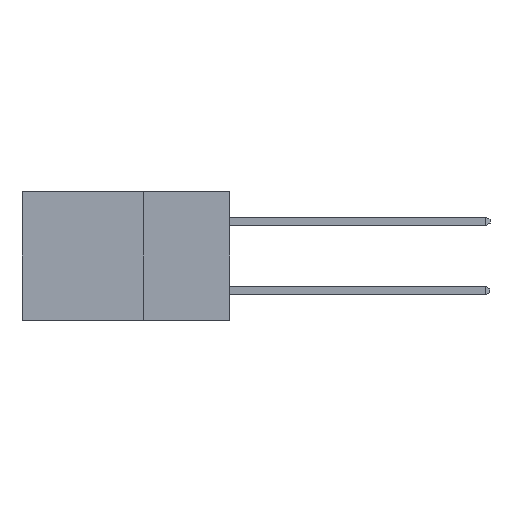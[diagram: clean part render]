
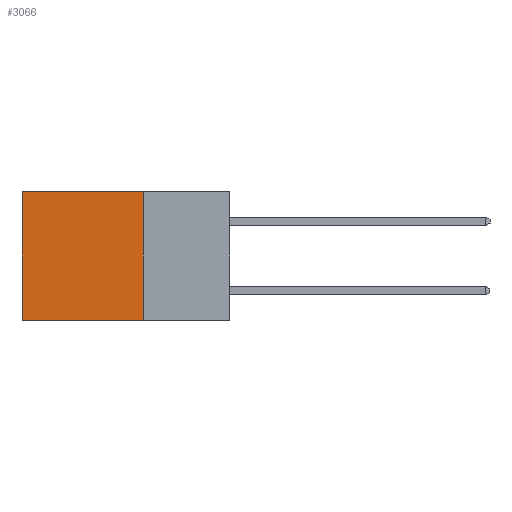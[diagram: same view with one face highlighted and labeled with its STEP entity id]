
A CAD part, left-side view. The second image highlights one B-rep face of the part: STEP entity #3066.
In plain terms, the highlighted planar face has unit normal (-1, 0, 0).
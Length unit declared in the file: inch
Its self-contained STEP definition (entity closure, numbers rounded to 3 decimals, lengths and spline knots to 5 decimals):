
#814 = AXIS2_PLACEMENT_3D ( 'NONE', #14183, #15251, #17469 ) ;
#2718 = VECTOR ( 'NONE', #5513, 39.37008 ) ;
#3066 = ADVANCED_FACE ( 'NONE', ( #17474 ), #12398, .F. ) ;
#3145 = VECTOR ( 'NONE', #8447, 39.37008 ) ;
#3818 = EDGE_CURVE ( 'NONE', #6233, #23538, #18302, .T. ) ;
#4454 = EDGE_CURVE ( 'NONE', #7965, #6233, #12601, .T. ) ;
#5513 = DIRECTION ( 'NONE',  ( 0., 0., -1. ) ) ;
#6233 = VERTEX_POINT ( 'NONE', #17590 ) ;
#7965 = VERTEX_POINT ( 'NONE', #8182 ) ;
#8182 = CARTESIAN_POINT ( 'NONE',  ( 0.298, 0.25, 0. ) ) ;
#8401 = ORIENTED_EDGE ( 'NONE', *, *, #19757, .F. ) ;
#8447 = DIRECTION ( 'NONE',  ( 0., 0., -1. ) ) ;
#8941 = EDGE_LOOP ( 'NONE', ( #13513, #8401, #20923, #21723 ) ) ;
#8965 = LINE ( 'NONE', #9352, #13860 ) ;
#9352 = CARTESIAN_POINT ( 'NONE',  ( 0.298, 0.25, -0.37 ) ) ;
#10825 = CARTESIAN_POINT ( 'NONE',  ( 0.298, 0.25, 0. ) ) ;
#10998 = VERTEX_POINT ( 'NONE', #14554 ) ;
#12398 = PLANE ( 'NONE',  #814 ) ;
#12601 = LINE ( 'NONE', #10825, #21585 ) ;
#13049 = DIRECTION ( 'NONE',  ( 0., 1., 0. ) ) ;
#13513 = ORIENTED_EDGE ( 'NONE', *, *, #3818, .T. ) ;
#13860 = VECTOR ( 'NONE', #13049, 39.37008 ) ;
#14183 = CARTESIAN_POINT ( 'NONE',  ( 0.298, 0.25, 0. ) ) ;
#14554 = CARTESIAN_POINT ( 'NONE',  ( 0.298, 0.25, -0.37 ) ) ;
#15251 = DIRECTION ( 'NONE',  ( 1., 0., 0. ) ) ;
#16837 = CARTESIAN_POINT ( 'NONE',  ( 0.298, 0.6, -0.37 ) ) ;
#17469 = DIRECTION ( 'NONE',  ( 0., 0., -1. ) ) ;
#17474 = FACE_OUTER_BOUND ( 'NONE', #8941, .T. ) ;
#17590 = CARTESIAN_POINT ( 'NONE',  ( 0.298, 0.6, 0. ) ) ;
#18189 = EDGE_CURVE ( 'NONE', #7965, #10998, #22027, .T. ) ;
#18302 = LINE ( 'NONE', #20590, #3145 ) ;
#19757 = EDGE_CURVE ( 'NONE', #10998, #23538, #8965, .T. ) ;
#20040 = CARTESIAN_POINT ( 'NONE',  ( 0.298, 0.25, 0. ) ) ;
#20590 = CARTESIAN_POINT ( 'NONE',  ( 0.298, 0.6, 0. ) ) ;
#20923 = ORIENTED_EDGE ( 'NONE', *, *, #18189, .F. ) ;
#21585 = VECTOR ( 'NONE', #22907, 39.37008 ) ;
#21723 = ORIENTED_EDGE ( 'NONE', *, *, #4454, .T. ) ;
#22027 = LINE ( 'NONE', #20040, #2718 ) ;
#22907 = DIRECTION ( 'NONE',  ( 0., 1., 0. ) ) ;
#23538 = VERTEX_POINT ( 'NONE', #16837 ) ;
